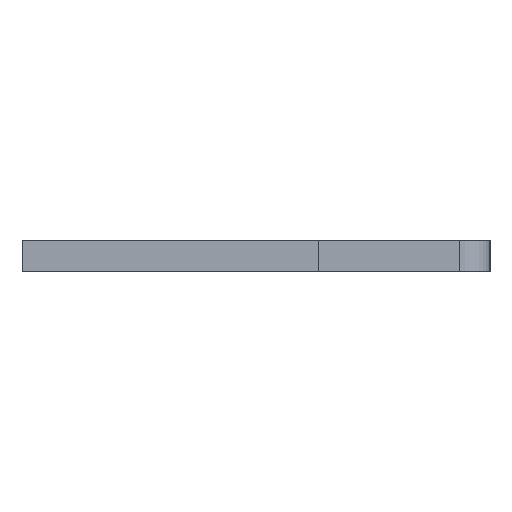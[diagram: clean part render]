
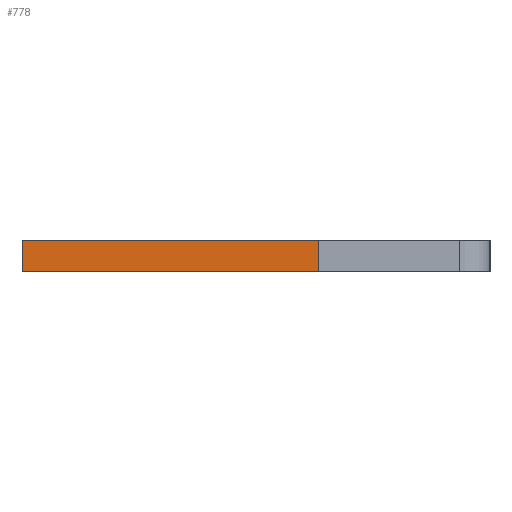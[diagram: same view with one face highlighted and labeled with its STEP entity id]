
A CAD part, left-side view. The second image highlights one B-rep face of the part: STEP entity #778.
In plain terms, the highlighted face is planar.
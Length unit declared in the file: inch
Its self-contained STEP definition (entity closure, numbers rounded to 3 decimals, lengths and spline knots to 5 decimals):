
#5 = CARTESIAN_POINT ( 'NONE',  ( -0.01, -0.04, -0.04 ) ) ;
#65 = CARTESIAN_POINT ( 'NONE',  ( 0.01, 0.15, -0.04 ) ) ;
#138 = DIRECTION ( 'NONE',  ( 0., 1., 0. ) ) ;
#153 = ORIENTED_EDGE ( 'NONE', *, *, #1975, .F. ) ;
#246 = VERTEX_POINT ( 'NONE', #531 ) ;
#276 = ORIENTED_EDGE ( 'NONE', *, *, #965, .T. ) ;
#321 = CARTESIAN_POINT ( 'NONE',  ( 0.01, -0.04, -0.04 ) ) ;
#343 = DIRECTION ( 'NONE',  ( -1., 0., 0. ) ) ;
#531 = CARTESIAN_POINT ( 'NONE',  ( -0.01, 0.15, -0.04 ) ) ;
#739 = VECTOR ( 'NONE', #804, 39.37008 ) ;
#741 = PLANE ( 'NONE',  #1948 ) ;
#778 = ADVANCED_FACE ( 'NONE', ( #1481 ), #741, .F. ) ;
#804 = DIRECTION ( 'NONE',  ( -1., 0., 0. ) ) ;
#821 = CARTESIAN_POINT ( 'NONE',  ( 0.01, 0.15, -0.04 ) ) ;
#856 = ORIENTED_EDGE ( 'NONE', *, *, #1460, .F. ) ;
#867 = VECTOR ( 'NONE', #343, 39.37008 ) ;
#904 = EDGE_LOOP ( 'NONE', ( #276, #153, #856, #1713 ) ) ;
#947 = VECTOR ( 'NONE', #2018, 39.37008 ) ;
#965 = EDGE_CURVE ( 'NONE', #1962, #246, #1335, .T. ) ;
#1075 = DIRECTION ( 'NONE',  ( 0., 0., 1. ) ) ;
#1152 = CARTESIAN_POINT ( 'NONE',  ( 0.01, -0.04, -0.04 ) ) ;
#1156 = LINE ( 'NONE', #321, #739 ) ;
#1202 = VECTOR ( 'NONE', #138, 39.37008 ) ;
#1252 = LINE ( 'NONE', #821, #867 ) ;
#1335 = LINE ( 'NONE', #1403, #947 ) ;
#1398 = DIRECTION ( 'NONE',  ( 1., 0., 0. ) ) ;
#1403 = CARTESIAN_POINT ( 'NONE',  ( -0.01, 0.15, -0.04 ) ) ;
#1460 = EDGE_CURVE ( 'NONE', #2067, #1857, #1512, .T. ) ;
#1481 = FACE_OUTER_BOUND ( 'NONE', #904, .T. ) ;
#1512 = LINE ( 'NONE', #1582, #1202 ) ;
#1582 = CARTESIAN_POINT ( 'NONE',  ( 0.01, 0.15, -0.04 ) ) ;
#1621 = CARTESIAN_POINT ( 'NONE',  ( 0.01, 0.15, -0.04 ) ) ;
#1713 = ORIENTED_EDGE ( 'NONE', *, *, #1721, .T. ) ;
#1721 = EDGE_CURVE ( 'NONE', #2067, #1962, #1156, .T. ) ;
#1857 = VERTEX_POINT ( 'NONE', #1621 ) ;
#1948 = AXIS2_PLACEMENT_3D ( 'NONE', #65, #1075, #1398 ) ;
#1962 = VERTEX_POINT ( 'NONE', #5 ) ;
#1975 = EDGE_CURVE ( 'NONE', #1857, #246, #1252, .T. ) ;
#2018 = DIRECTION ( 'NONE',  ( 0., 1., 0. ) ) ;
#2067 = VERTEX_POINT ( 'NONE', #1152 ) ;
